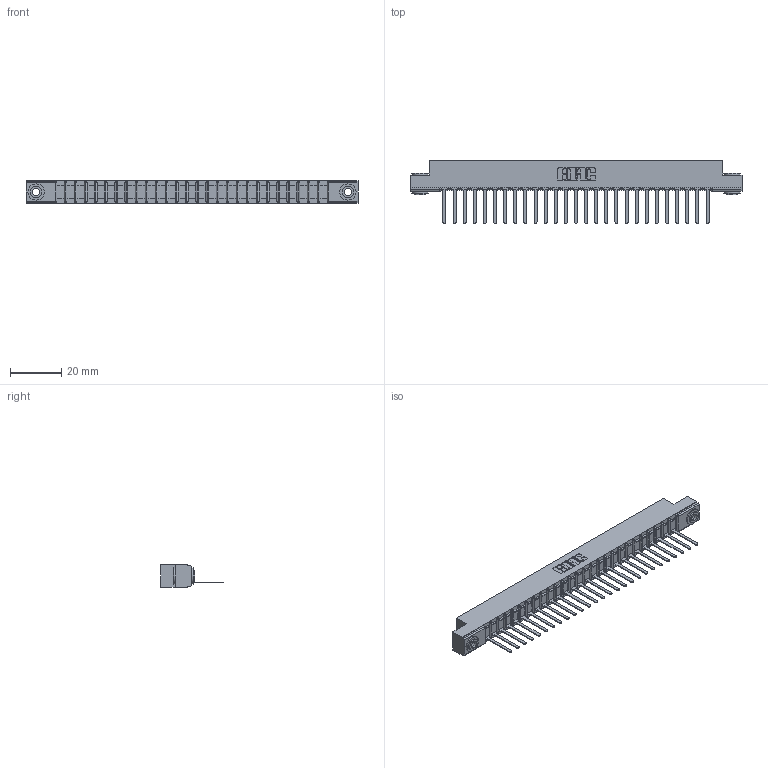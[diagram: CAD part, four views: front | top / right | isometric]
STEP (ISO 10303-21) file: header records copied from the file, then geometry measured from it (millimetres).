
FILE_DESCRIPTION (( 'STEP AP203' ), '1' );
FILE_NAME ('357-027-541-103.STEP', '2019-09-17T01:36:18', ( '' ), ( '' ), 'SwSTEP 2.0', 'SolidWorks 2016', '' );
FILE_SCHEMA (( 'CONFIG_CONTROL_DESIGN' ));
Length unit declared in the file: inch
Products named in the file (4): 357-027-541-103; 307 Part_.156 Dia Mounting Holes; 307-290-002_541; 345-250-002_345-250-002-102
Assembly tree (30 placements, depth 2):
  357-027-541-103
    307 Part_.156 Dia Mounting Holes
    307-290-002_541  x27
    345-250-002_345-250-002-102  x2
Bounding box: 130 x 24.59 x 8.71 mm (x, y, z)
Volume: 8662.3 mm3; surface area: 16737.3 mm2
Topology: 30 solids, 30 shells, 2196 faces, 6699 edges, 4386 vertices
Faces by surface type: plane 1309, cylinder 823, sphere 56, cone 8
Entity records: 26779 total; most frequent: CARTESIAN_POINT 4493, ORIENTED_EDGE 4474, DIRECTION 4387, EDGE_CURVE 2237, LINE 1699, VECTOR 1699, VERTEX_POINT 1450, AXIS2_PLACEMENT_3D 1344
